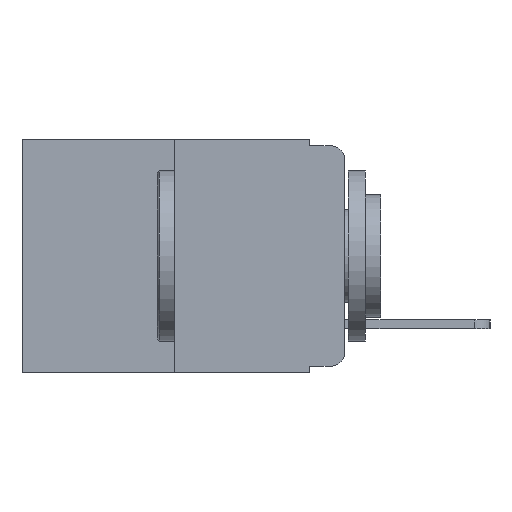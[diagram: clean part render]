
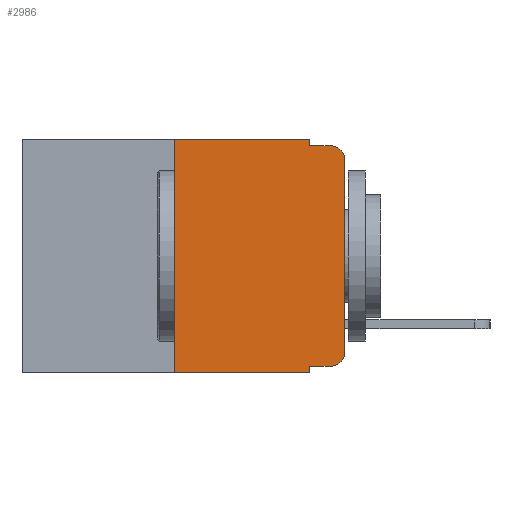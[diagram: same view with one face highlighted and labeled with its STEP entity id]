
A CAD part, left-side view. The second image highlights one B-rep face of the part: STEP entity #2986.
In plain terms, the highlighted planar face has unit normal (-1, 0, 0).
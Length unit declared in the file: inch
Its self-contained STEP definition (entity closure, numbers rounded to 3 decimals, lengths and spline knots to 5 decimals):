
#89 = EDGE_CURVE ( 'NONE', #7185, #18115, #7090, .T. ) ;
#257 = CARTESIAN_POINT ( 'NONE',  ( 0., 0.051, -0.343 ) ) ;
#454 = AXIS2_PLACEMENT_3D ( 'NONE', #7774, #18407, #9387 ) ;
#1251 = VERTEX_POINT ( 'NONE', #4553 ) ;
#1289 = CARTESIAN_POINT ( 'NONE',  ( 0., 0.051, -0.01 ) ) ;
#1293 = EDGE_CURVE ( 'NONE', #7185, #13595, #20651, .T. ) ;
#1326 = DIRECTION ( 'NONE',  ( 0., 0., -1. ) ) ;
#1375 = VERTEX_POINT ( 'NONE', #12054 ) ;
#1410 = ORIENTED_EDGE ( 'NONE', *, *, #2514, .F. ) ;
#1885 = ORIENTED_EDGE ( 'NONE', *, *, #1293, .F. ) ;
#2514 = EDGE_CURVE ( 'NONE', #4383, #12246, #13271, .T. ) ;
#2548 = CIRCLE ( 'NONE', #454, 0.02 ) ;
#2849 = CARTESIAN_POINT ( 'NONE',  ( 0., 0.02, -0.01 ) ) ;
#2986 = ADVANCED_FACE ( 'NONE', ( #4216 ), #9820, .F. ) ;
#3696 = CIRCLE ( 'NONE', #15606, 0.02 ) ;
#3874 = ORIENTED_EDGE ( 'NONE', *, *, #89, .T. ) ;
#4216 = FACE_OUTER_BOUND ( 'NONE', #9834, .T. ) ;
#4286 = VERTEX_POINT ( 'NONE', #1289 ) ;
#4329 = VECTOR ( 'NONE', #9509, 39.37008 ) ;
#4330 = ORIENTED_EDGE ( 'NONE', *, *, #10374, .T. ) ;
#4383 = VERTEX_POINT ( 'NONE', #6958 ) ;
#4409 = ORIENTED_EDGE ( 'NONE', *, *, #19827, .T. ) ;
#4553 = CARTESIAN_POINT ( 'NONE',  ( 0., 0., -0.313 ) ) ;
#4829 = ORIENTED_EDGE ( 'NONE', *, *, #7157, .F. ) ;
#5198 = EDGE_CURVE ( 'NONE', #12246, #20121, #16383, .T. ) ;
#5337 = VECTOR ( 'NONE', #12050, 39.37008 ) ;
#5340 = DIRECTION ( 'NONE',  ( 0., -1., 0. ) ) ;
#5492 = CARTESIAN_POINT ( 'NONE',  ( 0., 0.051, -0.333 ) ) ;
#6028 = EDGE_CURVE ( 'NONE', #20121, #4286, #12104, .T. ) ;
#6553 = CARTESIAN_POINT ( 'NONE',  ( 0., 0.473, 0. ) ) ;
#6958 = CARTESIAN_POINT ( 'NONE',  ( 0., 0.25, -0.343 ) ) ;
#7090 = LINE ( 'NONE', #9143, #14315 ) ;
#7157 = EDGE_CURVE ( 'NONE', #4286, #13966, #9092, .T. ) ;
#7185 = VERTEX_POINT ( 'NONE', #5492 ) ;
#7774 = CARTESIAN_POINT ( 'NONE',  ( 0., 0.02, -0.03 ) ) ;
#8189 = ORIENTED_EDGE ( 'NONE', *, *, #5198, .F. ) ;
#8610 = VECTOR ( 'NONE', #9104, 39.37008 ) ;
#8803 = VECTOR ( 'NONE', #18952, 39.37008 ) ;
#8844 = CARTESIAN_POINT ( 'NONE',  ( 0., 0.25, 0. ) ) ;
#8966 = CARTESIAN_POINT ( 'NONE',  ( 0., 0.02, -0.313 ) ) ;
#9092 = LINE ( 'NONE', #10238, #20661 ) ;
#9104 = DIRECTION ( 'NONE',  ( 0., 0., -1. ) ) ;
#9143 = CARTESIAN_POINT ( 'NONE',  ( 0., 0.051, -0.333 ) ) ;
#9338 = EDGE_CURVE ( 'NONE', #1375, #13966, #2548, .T. ) ;
#9353 = DIRECTION ( 'NONE',  ( 0., -1., 0. ) ) ;
#9387 = DIRECTION ( 'NONE',  ( 0., 0., -1. ) ) ;
#9509 = DIRECTION ( 'NONE',  ( 0., -1., 0. ) ) ;
#9820 = PLANE ( 'NONE',  #10009 ) ;
#9834 = EDGE_LOOP ( 'NONE', ( #4330, #13124, #4829, #11872, #8189, #1410, #10040, #1885, #3874, #4409 ) ) ;
#10009 = AXIS2_PLACEMENT_3D ( 'NONE', #6553, #11349, #1326 ) ;
#10040 = ORIENTED_EDGE ( 'NONE', *, *, #18686, .T. ) ;
#10238 = CARTESIAN_POINT ( 'NONE',  ( 0., 0.051, -0.01 ) ) ;
#10374 = EDGE_CURVE ( 'NONE', #1251, #1375, #19786, .T. ) ;
#10519 = DIRECTION ( 'NONE',  ( 0., 0., -1. ) ) ;
#10711 = CARTESIAN_POINT ( 'NONE',  ( 0., 0.051, 0. ) ) ;
#11349 = DIRECTION ( 'NONE',  ( 1., 0., 0. ) ) ;
#11643 = VECTOR ( 'NONE', #17008, 39.37008 ) ;
#11774 = VECTOR ( 'NONE', #20257, 39.37008 ) ;
#11872 = ORIENTED_EDGE ( 'NONE', *, *, #6028, .F. ) ;
#12050 = DIRECTION ( 'NONE',  ( 0., 0., 1. ) ) ;
#12054 = CARTESIAN_POINT ( 'NONE',  ( 0., 0., -0.03 ) ) ;
#12104 = LINE ( 'NONE', #10711, #11643 ) ;
#12246 = VERTEX_POINT ( 'NONE', #8844 ) ;
#13124 = ORIENTED_EDGE ( 'NONE', *, *, #9338, .T. ) ;
#13271 = LINE ( 'NONE', #13675, #5337 ) ;
#13595 = VERTEX_POINT ( 'NONE', #257 ) ;
#13675 = CARTESIAN_POINT ( 'NONE',  ( 0., 0.25, 0. ) ) ;
#13955 = CARTESIAN_POINT ( 'NONE',  ( 0., 0.051, 0. ) ) ;
#13966 = VERTEX_POINT ( 'NONE', #2849 ) ;
#14315 = VECTOR ( 'NONE', #9353, 39.37008 ) ;
#15166 = CARTESIAN_POINT ( 'NONE',  ( 0., 0.02, -0.333 ) ) ;
#15440 = CARTESIAN_POINT ( 'NONE',  ( 0., 0.051, 0. ) ) ;
#15606 = AXIS2_PLACEMENT_3D ( 'NONE', #8966, #19519, #10519 ) ;
#15919 = CARTESIAN_POINT ( 'NONE',  ( 0., 0.473, -0.343 ) ) ;
#16383 = LINE ( 'NONE', #20065, #4329 ) ;
#16816 = LINE ( 'NONE', #15919, #8803 ) ;
#17008 = DIRECTION ( 'NONE',  ( 0., 0., -1. ) ) ;
#17192 = CARTESIAN_POINT ( 'NONE',  ( 0., 0., 0. ) ) ;
#18115 = VERTEX_POINT ( 'NONE', #15166 ) ;
#18407 = DIRECTION ( 'NONE',  ( -1., 0., 0. ) ) ;
#18686 = EDGE_CURVE ( 'NONE', #4383, #13595, #16816, .T. ) ;
#18952 = DIRECTION ( 'NONE',  ( 0., -1., 0. ) ) ;
#19519 = DIRECTION ( 'NONE',  ( -1., 0., 0. ) ) ;
#19786 = LINE ( 'NONE', #17192, #11774 ) ;
#19827 = EDGE_CURVE ( 'NONE', #18115, #1251, #3696, .T. ) ;
#20065 = CARTESIAN_POINT ( 'NONE',  ( 0., 0.473, 0. ) ) ;
#20121 = VERTEX_POINT ( 'NONE', #13955 ) ;
#20257 = DIRECTION ( 'NONE',  ( 0., 0., 1. ) ) ;
#20651 = LINE ( 'NONE', #15440, #8610 ) ;
#20661 = VECTOR ( 'NONE', #5340, 39.37008 ) ;
